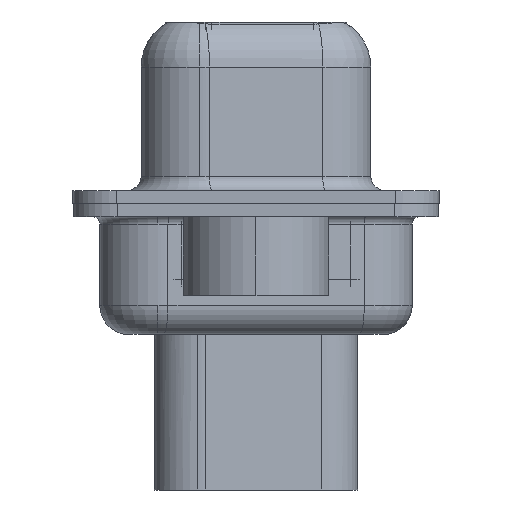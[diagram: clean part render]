
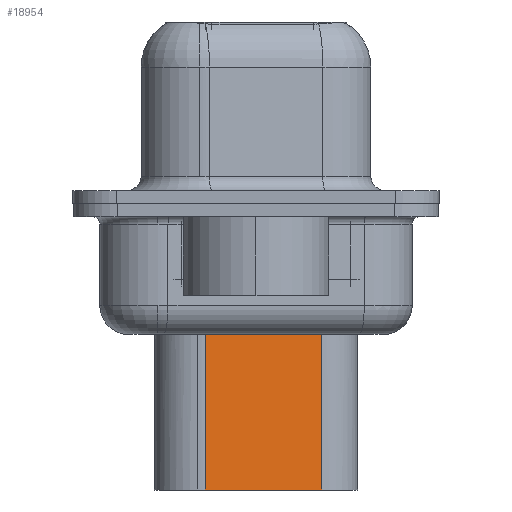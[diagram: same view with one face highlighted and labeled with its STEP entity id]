
A CAD part, left-side view. The second image highlights one B-rep face of the part: STEP entity #18954.
In plain terms, the highlighted planar face has unit normal (-0.985, -0.174, 0).
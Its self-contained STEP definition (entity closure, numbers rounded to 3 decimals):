
#1038 = ORIENTED_EDGE ( 'NONE', *, *, #2699, .T. ) ;
#1098 = CARTESIAN_POINT ( 'NONE',  ( 4.524, 1.74, -3.975 ) ) ;
#2196 = VERTEX_POINT ( 'NONE', #1098 ) ;
#2304 = EDGE_CURVE ( 'NONE', #20526, #2196, #20631, .T. ) ;
#2699 = EDGE_CURVE ( 'NONE', #2196, #26610, #15693, .T. ) ;
#3197 = CARTESIAN_POINT ( 'NONE',  ( 4.353, 2.709, -3.975 ) ) ;
#5029 = ORIENTED_EDGE ( 'NONE', *, *, #13514, .F. ) ;
#5778 = LINE ( 'NONE', #22870, #26429 ) ;
#7823 = EDGE_LOOP ( 'NONE', ( #5029, #8037, #1038, #30401 ) ) ;
#8037 = ORIENTED_EDGE ( 'NONE', *, *, #2304, .T. ) ;
#8174 = FACE_OUTER_BOUND ( 'NONE', #7823, .T. ) ;
#8442 = CARTESIAN_POINT ( 'NONE',  ( 4.524, 1.74, -3.1 ) ) ;
#8595 = DIRECTION ( 'NONE',  ( 0., 0., -1. ) ) ;
#8864 = DIRECTION ( 'NONE',  ( -0.174, 0.985, 0. ) ) ;
#13192 = EDGE_CURVE ( 'NONE', #17470, #26610, #28849, .T. ) ;
#13514 = EDGE_CURVE ( 'NONE', #20526, #17470, #5778, .T. ) ;
#13644 = DIRECTION ( 'NONE',  ( -0.985, -0.174, 0. ) ) ;
#15606 = VECTOR ( 'NONE', #8864, 1000. ) ;
#15693 = LINE ( 'NONE', #8442, #18460 ) ;
#16707 = CARTESIAN_POINT ( 'NONE',  ( 4.524, 1.74, -3.1 ) ) ;
#17470 = VERTEX_POINT ( 'NONE', #19643 ) ;
#18362 = DIRECTION ( 'NONE',  ( 0., 0., -1. ) ) ;
#18378 = DIRECTION ( 'NONE',  ( -0.174, 0.985, 0. ) ) ;
#18460 = VECTOR ( 'NONE', #8595, 1000. ) ;
#18954 = ADVANCED_FACE ( 'NONE', ( #8174 ), #23806, .T. ) ;
#19643 = CARTESIAN_POINT ( 'NONE',  ( 5.229, -2.26, -9.85 ) ) ;
#20526 = VERTEX_POINT ( 'NONE', #29610 ) ;
#20631 = LINE ( 'NONE', #3197, #20861 ) ;
#20861 = VECTOR ( 'NONE', #18378, 1000. ) ;
#21133 = CARTESIAN_POINT ( 'NONE',  ( 4.524, 1.74, -9.85 ) ) ;
#22870 = CARTESIAN_POINT ( 'NONE',  ( 5.229, -2.26, -3.1 ) ) ;
#23806 = PLANE ( 'NONE',  #29203 ) ;
#26286 = CARTESIAN_POINT ( 'NONE',  ( 4.524, 1.74, -9.85 ) ) ;
#26429 = VECTOR ( 'NONE', #18362, 1000. ) ;
#26610 = VERTEX_POINT ( 'NONE', #21133 ) ;
#28849 = LINE ( 'NONE', #26286, #15606 ) ;
#29203 = AXIS2_PLACEMENT_3D ( 'NONE', #16707, #13644, #31082 ) ;
#29610 = CARTESIAN_POINT ( 'NONE',  ( 5.229, -2.26, -3.975 ) ) ;
#30401 = ORIENTED_EDGE ( 'NONE', *, *, #13192, .F. ) ;
#31082 = DIRECTION ( 'NONE',  ( 0.174, -0.985, 0. ) ) ;
